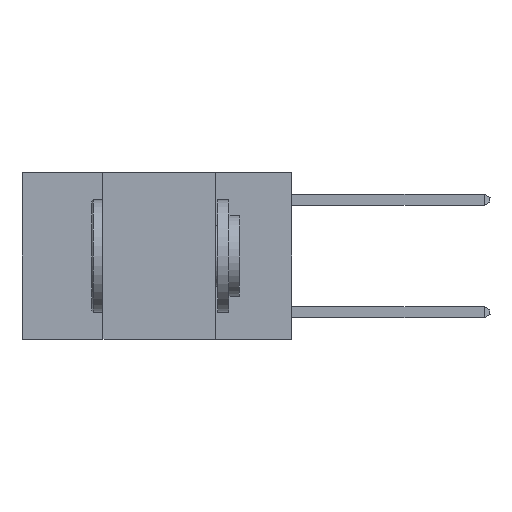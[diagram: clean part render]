
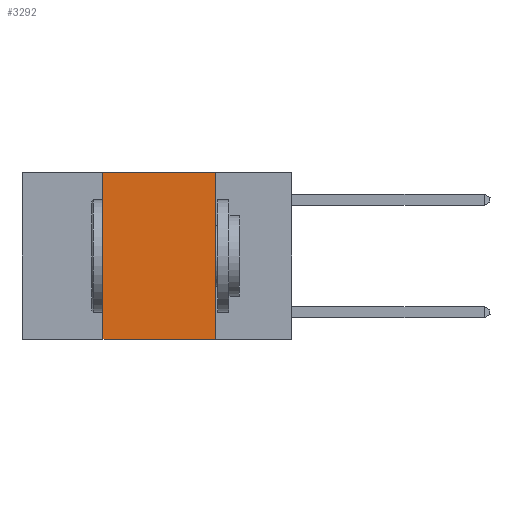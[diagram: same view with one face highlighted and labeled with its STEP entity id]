
A CAD part, left-side view. The second image highlights one B-rep face of the part: STEP entity #3292.
In plain terms, the highlighted planar face has unit normal (-1, 0, 0).
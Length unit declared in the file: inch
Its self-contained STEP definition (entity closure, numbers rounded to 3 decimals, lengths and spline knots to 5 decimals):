
#1106 = VERTEX_POINT ( 'NONE', #15990 ) ;
#1630 = CARTESIAN_POINT ( 'NONE',  ( 0., 0.17, -0.37 ) ) ;
#2549 = VERTEX_POINT ( 'NONE', #17180 ) ;
#2631 = DIRECTION ( 'NONE',  ( 1., 0., 0. ) ) ;
#3292 = ADVANCED_FACE ( 'NONE', ( #18691 ), #16694, .F. ) ;
#3364 = VECTOR ( 'NONE', #12547, 39.37008 ) ;
#3540 = ORIENTED_EDGE ( 'NONE', *, *, #20850, .F. ) ;
#4091 = VECTOR ( 'NONE', #18518, 39.37008 ) ;
#4510 = VECTOR ( 'NONE', #17768, 39.37008 ) ;
#5502 = CARTESIAN_POINT ( 'NONE',  ( 0., 0.42, 0. ) ) ;
#5605 = LINE ( 'NONE', #5502, #11243 ) ;
#5622 = CARTESIAN_POINT ( 'NONE',  ( 0., 0.6, 0. ) ) ;
#5767 = LINE ( 'NONE', #20366, #3364 ) ;
#6380 = LINE ( 'NONE', #14429, #4510 ) ;
#6615 = EDGE_CURVE ( 'NONE', #14541, #2549, #5605, .T. ) ;
#6811 = LINE ( 'NONE', #13276, #4091 ) ;
#9089 = EDGE_CURVE ( 'NONE', #1106, #13650, #6380, .T. ) ;
#9129 = DIRECTION ( 'NONE',  ( 0., 0., -1. ) ) ;
#10378 = DIRECTION ( 'NONE',  ( 0., 0., 1. ) ) ;
#11243 = VECTOR ( 'NONE', #10378, 39.37008 ) ;
#12547 = DIRECTION ( 'NONE',  ( 0., -1., 0. ) ) ;
#13276 = CARTESIAN_POINT ( 'NONE',  ( 0., 0.6, 0. ) ) ;
#13416 = AXIS2_PLACEMENT_3D ( 'NONE', #5622, #2631, #9129 ) ;
#13650 = VERTEX_POINT ( 'NONE', #1630 ) ;
#14429 = CARTESIAN_POINT ( 'NONE',  ( 0., 0.17, 0. ) ) ;
#14541 = VERTEX_POINT ( 'NONE', #17612 ) ;
#15440 = ORIENTED_EDGE ( 'NONE', *, *, #19190, .T. ) ;
#15990 = CARTESIAN_POINT ( 'NONE',  ( 0., 0.17, 0. ) ) ;
#16081 = ORIENTED_EDGE ( 'NONE', *, *, #9089, .F. ) ;
#16694 = PLANE ( 'NONE',  #13416 ) ;
#17180 = CARTESIAN_POINT ( 'NONE',  ( 0., 0.42, 0. ) ) ;
#17446 = EDGE_LOOP ( 'NONE', ( #16081, #3540, #20197, #15440 ) ) ;
#17612 = CARTESIAN_POINT ( 'NONE',  ( 0., 0.42, -0.37 ) ) ;
#17768 = DIRECTION ( 'NONE',  ( 0., 0., -1. ) ) ;
#18518 = DIRECTION ( 'NONE',  ( 0., -1., 0. ) ) ;
#18691 = FACE_OUTER_BOUND ( 'NONE', #17446, .T. ) ;
#19190 = EDGE_CURVE ( 'NONE', #14541, #13650, #5767, .T. ) ;
#20197 = ORIENTED_EDGE ( 'NONE', *, *, #6615, .F. ) ;
#20366 = CARTESIAN_POINT ( 'NONE',  ( 0., 0.6, -0.37 ) ) ;
#20850 = EDGE_CURVE ( 'NONE', #2549, #1106, #6811, .T. ) ;
